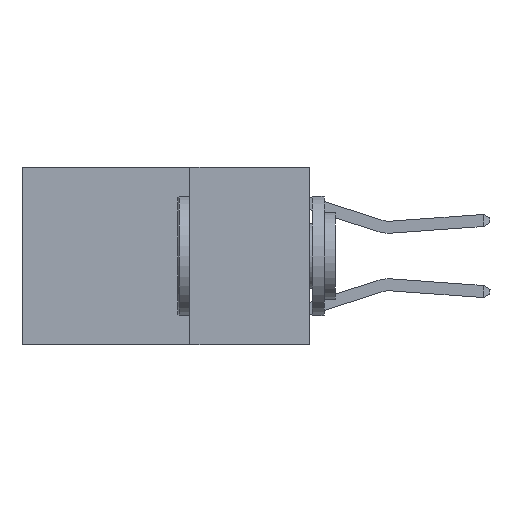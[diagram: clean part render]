
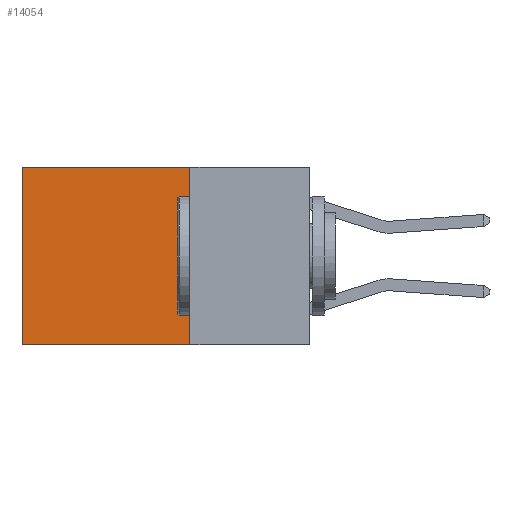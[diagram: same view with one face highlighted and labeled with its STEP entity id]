
A CAD part, left-side view. The second image highlights one B-rep face of the part: STEP entity #14054.
In plain terms, the highlighted planar face has unit normal (-1, 0, 0).
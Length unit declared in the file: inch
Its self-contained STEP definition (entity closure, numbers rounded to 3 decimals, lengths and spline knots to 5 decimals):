
#599 = DIRECTION ( 'NONE',  ( 0., 0., -1. ) ) ;
#600 = VECTOR ( 'NONE', #5791, 39.37008 ) ;
#1865 = DIRECTION ( 'NONE',  ( 0., 0., -1. ) ) ;
#1963 = LINE ( 'NONE', #19110, #12830 ) ;
#2069 = FACE_OUTER_BOUND ( 'NONE', #19192, .T. ) ;
#2497 = CARTESIAN_POINT ( 'NONE',  ( 0.2625, 0.6, 0. ) ) ;
#2750 = ORIENTED_EDGE ( 'NONE', *, *, #9237, .F. ) ;
#3134 = CARTESIAN_POINT ( 'NONE',  ( 0.2625, 0.25, 0. ) ) ;
#3313 = VECTOR ( 'NONE', #6729, 39.37008 ) ;
#3400 = EDGE_CURVE ( 'NONE', #8354, #14850, #7227, .T. ) ;
#4420 = CARTESIAN_POINT ( 'NONE',  ( 0.2625, 0.25, -0.37 ) ) ;
#5149 = DIRECTION ( 'NONE',  ( 1., 0., 0. ) ) ;
#5791 = DIRECTION ( 'NONE',  ( 0., 0., -1. ) ) ;
#6729 = DIRECTION ( 'NONE',  ( 0., 1., 0. ) ) ;
#6791 = ORIENTED_EDGE ( 'NONE', *, *, #3400, .T. ) ;
#6942 = AXIS2_PLACEMENT_3D ( 'NONE', #14594, #5149, #599 ) ;
#7227 = LINE ( 'NONE', #18422, #600 ) ;
#8121 = PLANE ( 'NONE',  #6942 ) ;
#8354 = VERTEX_POINT ( 'NONE', #2497 ) ;
#9237 = EDGE_CURVE ( 'NONE', #12466, #14850, #9951, .T. ) ;
#9837 = ORIENTED_EDGE ( 'NONE', *, *, #18355, .T. ) ;
#9951 = LINE ( 'NONE', #19203, #11160 ) ;
#11160 = VECTOR ( 'NONE', #14473, 39.37008 ) ;
#12200 = CARTESIAN_POINT ( 'NONE',  ( 0.2625, 0.6, -0.37 ) ) ;
#12466 = VERTEX_POINT ( 'NONE', #4420 ) ;
#12830 = VECTOR ( 'NONE', #1865, 39.37008 ) ;
#12906 = CARTESIAN_POINT ( 'NONE',  ( 0.2625, 0.25, 0. ) ) ;
#14054 = ADVANCED_FACE ( 'NONE', ( #2069 ), #8121, .F. ) ;
#14473 = DIRECTION ( 'NONE',  ( 0., 1., 0. ) ) ;
#14594 = CARTESIAN_POINT ( 'NONE',  ( 0.2625, 0.25, 0. ) ) ;
#14850 = VERTEX_POINT ( 'NONE', #12200 ) ;
#15660 = VERTEX_POINT ( 'NONE', #3134 ) ;
#15975 = LINE ( 'NONE', #12906, #3313 ) ;
#16589 = ORIENTED_EDGE ( 'NONE', *, *, #17854, .F. ) ;
#17854 = EDGE_CURVE ( 'NONE', #15660, #12466, #1963, .T. ) ;
#18355 = EDGE_CURVE ( 'NONE', #15660, #8354, #15975, .T. ) ;
#18422 = CARTESIAN_POINT ( 'NONE',  ( 0.2625, 0.6, 0. ) ) ;
#19110 = CARTESIAN_POINT ( 'NONE',  ( 0.2625, 0.25, 0. ) ) ;
#19192 = EDGE_LOOP ( 'NONE', ( #6791, #2750, #16589, #9837 ) ) ;
#19203 = CARTESIAN_POINT ( 'NONE',  ( 0.2625, 0.25, -0.37 ) ) ;
